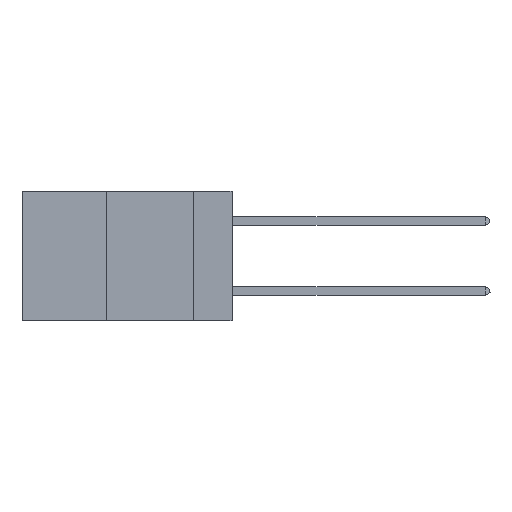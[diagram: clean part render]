
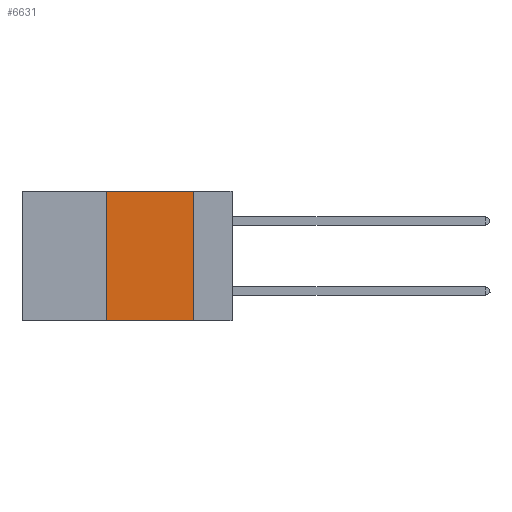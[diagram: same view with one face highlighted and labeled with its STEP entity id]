
A CAD part, left-side view. The second image highlights one B-rep face of the part: STEP entity #6631.
In plain terms, the highlighted planar face has unit normal (-1, 0, 0).
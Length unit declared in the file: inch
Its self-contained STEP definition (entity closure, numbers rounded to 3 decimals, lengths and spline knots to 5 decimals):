
#226 = LINE ( 'NONE', #15378, #13908 ) ;
#474 = VERTEX_POINT ( 'NONE', #5520 ) ;
#492 = DIRECTION ( 'NONE',  ( 0., -1., 0. ) ) ;
#581 = VERTEX_POINT ( 'NONE', #14084 ) ;
#667 = DIRECTION ( 'NONE',  ( 0., 0., -1. ) ) ;
#1374 = ORIENTED_EDGE ( 'NONE', *, *, #1557, .F. ) ;
#1557 = EDGE_CURVE ( 'NONE', #10477, #474, #10980, .T. ) ;
#2193 = DIRECTION ( 'NONE',  ( 0., -1., 0. ) ) ;
#2606 = EDGE_CURVE ( 'NONE', #13047, #581, #3555, .T. ) ;
#3555 = LINE ( 'NONE', #16576, #11557 ) ;
#3803 = DIRECTION ( 'NONE',  ( 1., 0., 0. ) ) ;
#4625 = CARTESIAN_POINT ( 'NONE',  ( 0., 0.6, 0. ) ) ;
#5520 = CARTESIAN_POINT ( 'NONE',  ( 0., 0.11, 0. ) ) ;
#5744 = AXIS2_PLACEMENT_3D ( 'NONE', #4625, #3803, #9189 ) ;
#6212 = ORIENTED_EDGE ( 'NONE', *, *, #14028, .F. ) ;
#6424 = CARTESIAN_POINT ( 'NONE',  ( 0., 0.36, -0.37 ) ) ;
#6631 = ADVANCED_FACE ( 'NONE', ( #9242 ), #8112, .F. ) ;
#7565 = CARTESIAN_POINT ( 'NONE',  ( 0., 0.6, 0. ) ) ;
#8112 = PLANE ( 'NONE',  #5744 ) ;
#9189 = DIRECTION ( 'NONE',  ( 0., 0., -1. ) ) ;
#9242 = FACE_OUTER_BOUND ( 'NONE', #15335, .T. ) ;
#9710 = VECTOR ( 'NONE', #2193, 39.37008 ) ;
#9994 = VECTOR ( 'NONE', #10041, 39.37008 ) ;
#10041 = DIRECTION ( 'NONE',  ( 0., 0., 1. ) ) ;
#10398 = CARTESIAN_POINT ( 'NONE',  ( 0., 0.36, 0. ) ) ;
#10477 = VERTEX_POINT ( 'NONE', #10398 ) ;
#10980 = LINE ( 'NONE', #7565, #9710 ) ;
#11324 = CARTESIAN_POINT ( 'NONE',  ( 0., 0.36, 0. ) ) ;
#11557 = VECTOR ( 'NONE', #492, 39.37008 ) ;
#13047 = VERTEX_POINT ( 'NONE', #6424 ) ;
#13286 = ORIENTED_EDGE ( 'NONE', *, *, #2606, .T. ) ;
#13908 = VECTOR ( 'NONE', #667, 39.37008 ) ;
#14028 = EDGE_CURVE ( 'NONE', #13047, #10477, #16660, .T. ) ;
#14084 = CARTESIAN_POINT ( 'NONE',  ( 0., 0.11, -0.37 ) ) ;
#15089 = EDGE_CURVE ( 'NONE', #474, #581, #226, .T. ) ;
#15335 = EDGE_LOOP ( 'NONE', ( #17370, #1374, #6212, #13286 ) ) ;
#15378 = CARTESIAN_POINT ( 'NONE',  ( 0., 0.11, 0. ) ) ;
#16576 = CARTESIAN_POINT ( 'NONE',  ( 0., 0.6, -0.37 ) ) ;
#16660 = LINE ( 'NONE', #11324, #9994 ) ;
#17370 = ORIENTED_EDGE ( 'NONE', *, *, #15089, .F. ) ;
